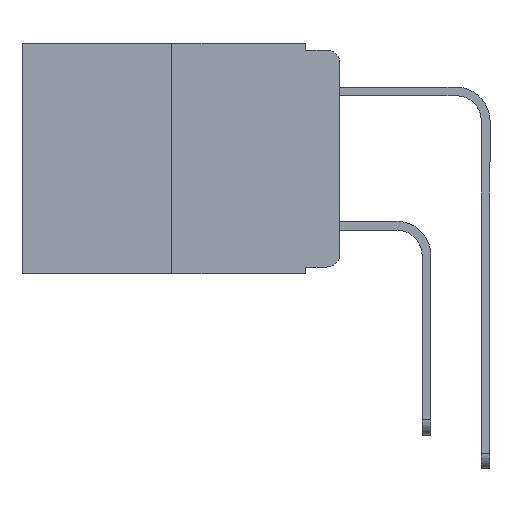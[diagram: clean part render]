
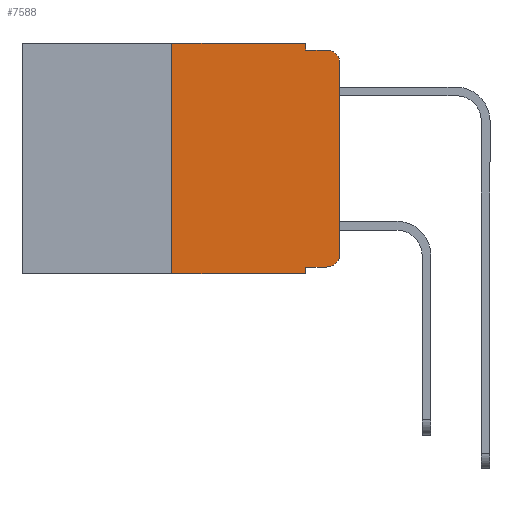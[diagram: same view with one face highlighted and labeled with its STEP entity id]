
A CAD part, left-side view. The second image highlights one B-rep face of the part: STEP entity #7588.
In plain terms, the highlighted planar face has unit normal (-1, 0, 0).
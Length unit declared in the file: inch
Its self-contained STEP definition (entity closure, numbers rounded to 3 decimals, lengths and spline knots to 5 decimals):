
#87 = CARTESIAN_POINT ( 'NONE',  ( 0., 0.02, -0.03 ) ) ;
#88 = ORIENTED_EDGE ( 'NONE', *, *, #9146, .T. ) ;
#175 = VECTOR ( 'NONE', #3713, 39.37008 ) ;
#563 = ORIENTED_EDGE ( 'NONE', *, *, #12069, .T. ) ;
#710 = EDGE_CURVE ( 'NONE', #1372, #11394, #12081, .T. ) ;
#870 = CARTESIAN_POINT ( 'NONE',  ( 0., 0.051, -0.01 ) ) ;
#981 = ORIENTED_EDGE ( 'NONE', *, *, #8517, .T. ) ;
#1024 = VECTOR ( 'NONE', #2976, 39.37008 ) ;
#1171 = DIRECTION ( 'NONE',  ( 0., 0., -1. ) ) ;
#1187 = LINE ( 'NONE', #9234, #3731 ) ;
#1200 = ORIENTED_EDGE ( 'NONE', *, *, #10244, .F. ) ;
#1205 = DIRECTION ( 'NONE',  ( 0., -1., 0. ) ) ;
#1322 = LINE ( 'NONE', #7644, #1024 ) ;
#1372 = VERTEX_POINT ( 'NONE', #12005 ) ;
#1499 = VERTEX_POINT ( 'NONE', #6156 ) ;
#1582 = AXIS2_PLACEMENT_3D ( 'NONE', #3223, #9709, #4191 ) ;
#1696 = CIRCLE ( 'NONE', #1582, 0.02 ) ;
#1719 = LINE ( 'NONE', #6451, #10972 ) ;
#1788 = EDGE_CURVE ( 'NONE', #2509, #1876, #1719, .T. ) ;
#1876 = VERTEX_POINT ( 'NONE', #2645 ) ;
#2115 = ORIENTED_EDGE ( 'NONE', *, *, #1788, .T. ) ;
#2187 = CARTESIAN_POINT ( 'NONE',  ( 0., 0.051, -0.333 ) ) ;
#2218 = EDGE_LOOP ( 'NONE', ( #8267, #563, #5649, #5933, #1200, #6542, #2115, #9537, #88, #981 ) ) ;
#2393 = CARTESIAN_POINT ( 'NONE',  ( 0., 0.051, 0. ) ) ;
#2509 = VERTEX_POINT ( 'NONE', #6662 ) ;
#2534 = LINE ( 'NONE', #870, #175 ) ;
#2645 = CARTESIAN_POINT ( 'NONE',  ( 0., 0.051, -0.343 ) ) ;
#2789 = CARTESIAN_POINT ( 'NONE',  ( 0., 0.25, 0. ) ) ;
#2848 = VECTOR ( 'NONE', #10170, 39.37008 ) ;
#2976 = DIRECTION ( 'NONE',  ( 0., 0., -1. ) ) ;
#3223 = CARTESIAN_POINT ( 'NONE',  ( 0., 0.02, -0.313 ) ) ;
#3565 = AXIS2_PLACEMENT_3D ( 'NONE', #8977, #5258, #5297 ) ;
#3639 = CARTESIAN_POINT ( 'NONE',  ( 0., 0.02, -0.01 ) ) ;
#3713 = DIRECTION ( 'NONE',  ( 0., -1., 0. ) ) ;
#3731 = VECTOR ( 'NONE', #10098, 39.37008 ) ;
#4191 = DIRECTION ( 'NONE',  ( 0., 0., -1. ) ) ;
#4289 = CARTESIAN_POINT ( 'NONE',  ( 0., 0., 0. ) ) ;
#4349 = LINE ( 'NONE', #5794, #11323 ) ;
#4364 = PLANE ( 'NONE',  #3565 ) ;
#4596 = VECTOR ( 'NONE', #10373, 39.37008 ) ;
#5258 = DIRECTION ( 'NONE',  ( 1., 0., 0. ) ) ;
#5297 = DIRECTION ( 'NONE',  ( 0., 0., -1. ) ) ;
#5354 = LINE ( 'NONE', #2789, #2848 ) ;
#5521 = LINE ( 'NONE', #2187, #10661 ) ;
#5558 = DIRECTION ( 'NONE',  ( 0., -1., 0. ) ) ;
#5649 = ORIENTED_EDGE ( 'NONE', *, *, #11487, .F. ) ;
#5794 = CARTESIAN_POINT ( 'NONE',  ( 0., 0.051, 0. ) ) ;
#5803 = CARTESIAN_POINT ( 'NONE',  ( 0., 0.02, -0.333 ) ) ;
#5933 = ORIENTED_EDGE ( 'NONE', *, *, #10925, .F. ) ;
#6028 = VERTEX_POINT ( 'NONE', #2393 ) ;
#6156 = CARTESIAN_POINT ( 'NONE',  ( 0., 0.051, -0.333 ) ) ;
#6451 = CARTESIAN_POINT ( 'NONE',  ( 0., 0.473, -0.343 ) ) ;
#6542 = ORIENTED_EDGE ( 'NONE', *, *, #10310, .F. ) ;
#6662 = CARTESIAN_POINT ( 'NONE',  ( 0., 0.25, -0.343 ) ) ;
#6690 = CARTESIAN_POINT ( 'NONE',  ( 0., 0.051, -0.01 ) ) ;
#6843 = DIRECTION ( 'NONE',  ( -1., 0., 0. ) ) ;
#6863 = VERTEX_POINT ( 'NONE', #8991 ) ;
#7291 = CARTESIAN_POINT ( 'NONE',  ( 0., 0., -0.03 ) ) ;
#7588 = ADVANCED_FACE ( 'NONE', ( #9183 ), #4364, .F. ) ;
#7644 = CARTESIAN_POINT ( 'NONE',  ( 0., 0.051, 0. ) ) ;
#8267 = ORIENTED_EDGE ( 'NONE', *, *, #710, .T. ) ;
#8373 = VERTEX_POINT ( 'NONE', #3639 ) ;
#8517 = EDGE_CURVE ( 'NONE', #9042, #1372, #1696, .T. ) ;
#8977 = CARTESIAN_POINT ( 'NONE',  ( 0., 0.473, 0. ) ) ;
#8991 = CARTESIAN_POINT ( 'NONE',  ( 0., 0.25, 0. ) ) ;
#9042 = VERTEX_POINT ( 'NONE', #5803 ) ;
#9146 = EDGE_CURVE ( 'NONE', #1499, #9042, #5521, .T. ) ;
#9183 = FACE_OUTER_BOUND ( 'NONE', #2218, .T. ) ;
#9234 = CARTESIAN_POINT ( 'NONE',  ( 0., 0.473, 0. ) ) ;
#9458 = DIRECTION ( 'NONE',  ( 0., 0., -1. ) ) ;
#9537 = ORIENTED_EDGE ( 'NONE', *, *, #9726, .F. ) ;
#9709 = DIRECTION ( 'NONE',  ( -1., 0., 0. ) ) ;
#9726 = EDGE_CURVE ( 'NONE', #1499, #1876, #4349, .T. ) ;
#10013 = AXIS2_PLACEMENT_3D ( 'NONE', #87, #6843, #1171 ) ;
#10098 = DIRECTION ( 'NONE',  ( 0., -1., 0. ) ) ;
#10170 = DIRECTION ( 'NONE',  ( 0., 0., 1. ) ) ;
#10244 = EDGE_CURVE ( 'NONE', #6863, #6028, #1187, .T. ) ;
#10310 = EDGE_CURVE ( 'NONE', #2509, #6863, #5354, .T. ) ;
#10373 = DIRECTION ( 'NONE',  ( 0., 0., 1. ) ) ;
#10602 = CIRCLE ( 'NONE', #10013, 0.02 ) ;
#10661 = VECTOR ( 'NONE', #1205, 39.37008 ) ;
#10925 = EDGE_CURVE ( 'NONE', #6028, #11991, #1322, .T. ) ;
#10972 = VECTOR ( 'NONE', #5558, 39.37008 ) ;
#11323 = VECTOR ( 'NONE', #9458, 39.37008 ) ;
#11394 = VERTEX_POINT ( 'NONE', #7291 ) ;
#11487 = EDGE_CURVE ( 'NONE', #11991, #8373, #2534, .T. ) ;
#11991 = VERTEX_POINT ( 'NONE', #6690 ) ;
#12005 = CARTESIAN_POINT ( 'NONE',  ( 0., 0., -0.313 ) ) ;
#12069 = EDGE_CURVE ( 'NONE', #11394, #8373, #10602, .T. ) ;
#12081 = LINE ( 'NONE', #4289, #4596 ) ;
